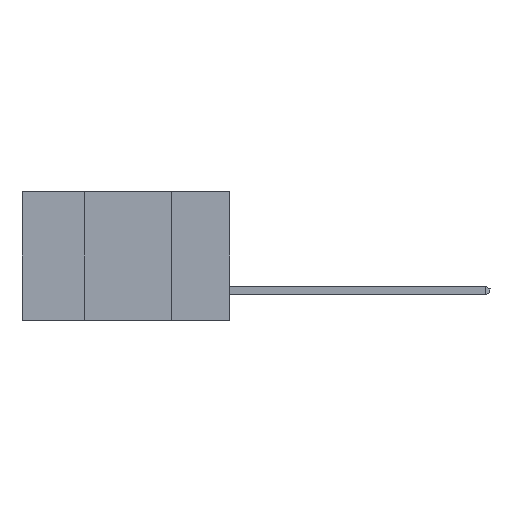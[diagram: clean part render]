
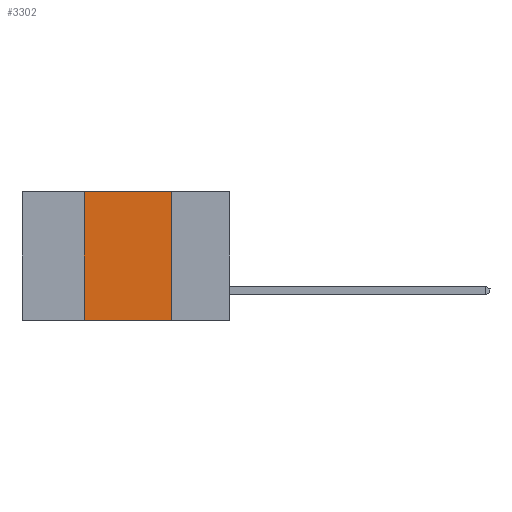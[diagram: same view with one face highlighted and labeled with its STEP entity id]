
A CAD part, left-side view. The second image highlights one B-rep face of the part: STEP entity #3302.
In plain terms, the highlighted planar face has unit normal (-1, 0, 0).
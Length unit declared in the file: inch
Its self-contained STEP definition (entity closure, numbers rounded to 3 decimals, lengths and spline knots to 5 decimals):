
#11 = DIRECTION ( 'NONE',  ( 0., 0., -1. ) ) ;
#1159 = ORIENTED_EDGE ( 'NONE', *, *, #19180, .T. ) ;
#1344 = ORIENTED_EDGE ( 'NONE', *, *, #14359, .F. ) ;
#3302 = ADVANCED_FACE ( 'NONE', ( #4521 ), #17729, .F. ) ;
#4450 = DIRECTION ( 'NONE',  ( 0., -1., 0. ) ) ;
#4521 = FACE_OUTER_BOUND ( 'NONE', #10737, .T. ) ;
#5330 = AXIS2_PLACEMENT_3D ( 'NONE', #6791, #14212, #10291 ) ;
#5779 = CARTESIAN_POINT ( 'NONE',  ( 0., 0.17, -0.37 ) ) ;
#6791 = CARTESIAN_POINT ( 'NONE',  ( 0., 0.6, 0. ) ) ;
#6801 = VERTEX_POINT ( 'NONE', #20071 ) ;
#7245 = ORIENTED_EDGE ( 'NONE', *, *, #18379, .F. ) ;
#8027 = ORIENTED_EDGE ( 'NONE', *, *, #14361, .F. ) ;
#9561 = LINE ( 'NONE', #5779, #13508 ) ;
#10291 = DIRECTION ( 'NONE',  ( 0., 0., -1. ) ) ;
#10677 = VECTOR ( 'NONE', #23047, 39.37008 ) ;
#10737 = EDGE_LOOP ( 'NONE', ( #1344, #8027, #7245, #1159 ) ) ;
#11567 = CARTESIAN_POINT ( 'NONE',  ( 0., 0.6, 0. ) ) ;
#11647 = VERTEX_POINT ( 'NONE', #16606 ) ;
#11810 = DIRECTION ( 'NONE',  ( 0., 0., 1. ) ) ;
#13139 = CARTESIAN_POINT ( 'NONE',  ( 0., 0.42, 0. ) ) ;
#13453 = LINE ( 'NONE', #11567, #10677 ) ;
#13508 = VECTOR ( 'NONE', #11, 39.37008 ) ;
#13702 = LINE ( 'NONE', #21381, #16060 ) ;
#14212 = DIRECTION ( 'NONE',  ( 1., 0., 0. ) ) ;
#14359 = EDGE_CURVE ( 'NONE', #21508, #11647, #9561, .T. ) ;
#14361 = EDGE_CURVE ( 'NONE', #22804, #21508, #13453, .T. ) ;
#15033 = CARTESIAN_POINT ( 'NONE',  ( 0., 0.17, 0. ) ) ;
#15296 = VECTOR ( 'NONE', #4450, 39.37008 ) ;
#16060 = VECTOR ( 'NONE', #11810, 39.37008 ) ;
#16606 = CARTESIAN_POINT ( 'NONE',  ( 0., 0.17, -0.37 ) ) ;
#17729 = PLANE ( 'NONE',  #5330 ) ;
#18379 = EDGE_CURVE ( 'NONE', #6801, #22804, #13702, .T. ) ;
#19180 = EDGE_CURVE ( 'NONE', #6801, #11647, #23721, .T. ) ;
#20071 = CARTESIAN_POINT ( 'NONE',  ( 0., 0.42, -0.37 ) ) ;
#21381 = CARTESIAN_POINT ( 'NONE',  ( 0., 0.42, -0.37 ) ) ;
#21508 = VERTEX_POINT ( 'NONE', #15033 ) ;
#21700 = CARTESIAN_POINT ( 'NONE',  ( 0., 0.6, -0.37 ) ) ;
#22804 = VERTEX_POINT ( 'NONE', #13139 ) ;
#23047 = DIRECTION ( 'NONE',  ( 0., -1., 0. ) ) ;
#23721 = LINE ( 'NONE', #21700, #15296 ) ;
